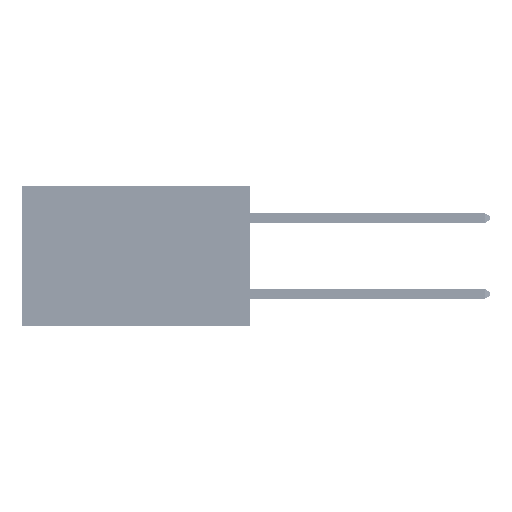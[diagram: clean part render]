
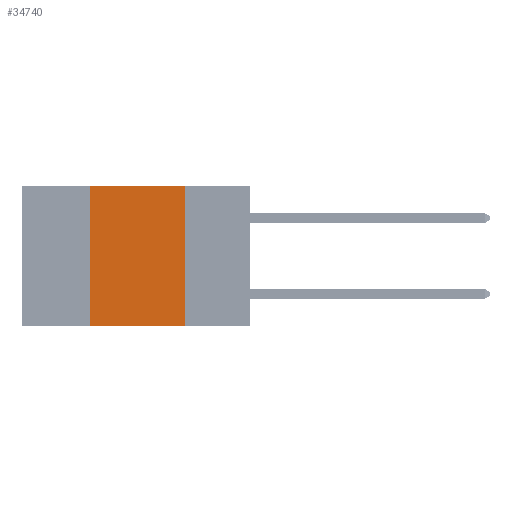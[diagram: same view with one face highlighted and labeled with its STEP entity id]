
A CAD part, left-side view. The second image highlights one B-rep face of the part: STEP entity #34740.
In plain terms, the highlighted planar face has unit normal (-1, 0, 0).
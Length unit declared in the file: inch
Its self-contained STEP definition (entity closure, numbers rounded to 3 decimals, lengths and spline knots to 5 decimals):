
#2926 = VECTOR ( 'NONE', #30332, 39.37008 ) ;
#3869 = CARTESIAN_POINT ( 'NONE',  ( 0., 0.6, -0.37 ) ) ;
#4356 = DIRECTION ( 'NONE',  ( 0., 0., -1. ) ) ;
#7297 = AXIS2_PLACEMENT_3D ( 'NONE', #10384, #36973, #14271 ) ;
#10103 = ORIENTED_EDGE ( 'NONE', *, *, #16658, .T. ) ;
#10384 = CARTESIAN_POINT ( 'NONE',  ( 0., 0.6, 0. ) ) ;
#11241 = ORIENTED_EDGE ( 'NONE', *, *, #37427, .F. ) ;
#11347 = CARTESIAN_POINT ( 'NONE',  ( 0., 0.6, 0. ) ) ;
#11700 = EDGE_LOOP ( 'NONE', ( #12005, #11241, #19637, #10103 ) ) ;
#11715 = VERTEX_POINT ( 'NONE', #36364 ) ;
#12005 = ORIENTED_EDGE ( 'NONE', *, *, #40128, .F. ) ;
#14271 = DIRECTION ( 'NONE',  ( 0., 0., -1. ) ) ;
#16024 = CARTESIAN_POINT ( 'NONE',  ( 0., 0.17, 0. ) ) ;
#16658 = EDGE_CURVE ( 'NONE', #33674, #32928, #43996, .T. ) ;
#17100 = CARTESIAN_POINT ( 'NONE',  ( 0., 0.17, -0.37 ) ) ;
#19227 = VERTEX_POINT ( 'NONE', #48121 ) ;
#19637 = ORIENTED_EDGE ( 'NONE', *, *, #47894, .F. ) ;
#20223 = LINE ( 'NONE', #16024, #39143 ) ;
#21110 = CARTESIAN_POINT ( 'NONE',  ( 0., 0.42, 0. ) ) ;
#21777 = PLANE ( 'NONE',  #7297 ) ;
#24626 = LINE ( 'NONE', #11347, #2926 ) ;
#25811 = FACE_OUTER_BOUND ( 'NONE', #11700, .T. ) ;
#28746 = DIRECTION ( 'NONE',  ( 0., 0., 1. ) ) ;
#30145 = LINE ( 'NONE', #21110, #41310 ) ;
#30332 = DIRECTION ( 'NONE',  ( 0., -1., 0. ) ) ;
#32628 = CARTESIAN_POINT ( 'NONE',  ( 0., 0.42, -0.37 ) ) ;
#32928 = VERTEX_POINT ( 'NONE', #17100 ) ;
#33674 = VERTEX_POINT ( 'NONE', #32628 ) ;
#34740 = ADVANCED_FACE ( 'NONE', ( #25811 ), #21777, .F. ) ;
#36364 = CARTESIAN_POINT ( 'NONE',  ( 0., 0.42, 0. ) ) ;
#36973 = DIRECTION ( 'NONE',  ( 1., 0., 0. ) ) ;
#37427 = EDGE_CURVE ( 'NONE', #11715, #19227, #24626, .T. ) ;
#39143 = VECTOR ( 'NONE', #4356, 39.37008 ) ;
#40128 = EDGE_CURVE ( 'NONE', #19227, #32928, #20223, .T. ) ;
#41310 = VECTOR ( 'NONE', #28746, 39.37008 ) ;
#43996 = LINE ( 'NONE', #3869, #45168 ) ;
#45168 = VECTOR ( 'NONE', #45578, 39.37008 ) ;
#45578 = DIRECTION ( 'NONE',  ( 0., -1., 0. ) ) ;
#47894 = EDGE_CURVE ( 'NONE', #33674, #11715, #30145, .T. ) ;
#48121 = CARTESIAN_POINT ( 'NONE',  ( 0., 0.17, 0. ) ) ;
